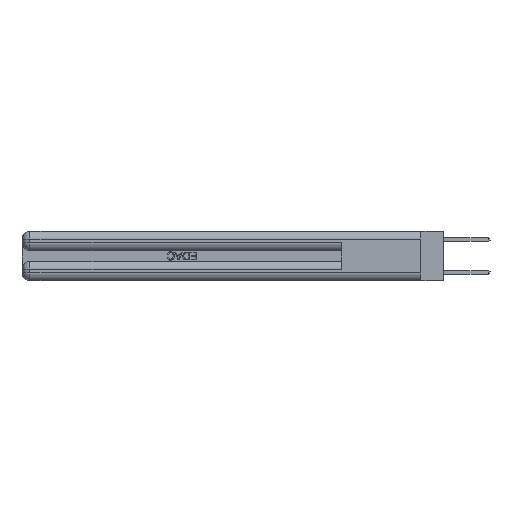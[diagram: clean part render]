
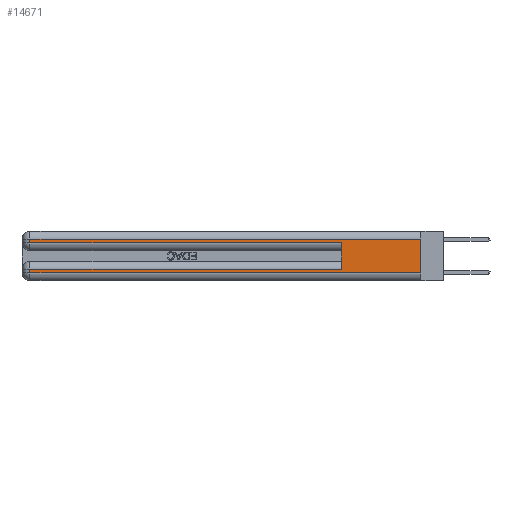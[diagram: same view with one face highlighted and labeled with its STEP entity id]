
A CAD part, left-side view. The second image highlights one B-rep face of the part: STEP entity #14671.
In plain terms, the highlighted planar face has unit normal (-1, 0, 0).
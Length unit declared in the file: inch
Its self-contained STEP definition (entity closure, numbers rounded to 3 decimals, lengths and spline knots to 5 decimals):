
#232 = CARTESIAN_POINT ( 'NONE',  ( 0., 0., 0.31 ) ) ;
#868 = CARTESIAN_POINT ( 'NONE',  ( 0., 0., 0.37 ) ) ;
#1439 = CARTESIAN_POINT ( 'NONE',  ( 0., 0.6, 0.145 ) ) ;
#1994 = CARTESIAN_POINT ( 'NONE',  ( 0., 2.94, 0.37 ) ) ;
#2072 = ORIENTED_EDGE ( 'NONE', *, *, #24333, .T. ) ;
#3748 = DIRECTION ( 'NONE',  ( 1., 0., 0. ) ) ;
#3786 = DIRECTION ( 'NONE',  ( 0., 1., 0. ) ) ;
#4033 = VECTOR ( 'NONE', #19386, 39.37008 ) ;
#4073 = VECTOR ( 'NONE', #12754, 39.37008 ) ;
#4190 = CARTESIAN_POINT ( 'NONE',  ( 0., 0.6, 0.285 ) ) ;
#4541 = VERTEX_POINT ( 'NONE', #232 ) ;
#4792 = EDGE_CURVE ( 'NONE', #25713, #32204, #33472, .T. ) ;
#4947 = CARTESIAN_POINT ( 'NONE',  ( 0., 0., 0.285 ) ) ;
#5174 = VERTEX_POINT ( 'NONE', #31147 ) ;
#5630 = FACE_OUTER_BOUND ( 'NONE', #18114, .T. ) ;
#5877 = LINE ( 'NONE', #23058, #18898 ) ;
#6047 = CARTESIAN_POINT ( 'NONE',  ( 0., 2.94, 0.37 ) ) ;
#7306 = ORIENTED_EDGE ( 'NONE', *, *, #11483, .T. ) ;
#7580 = DIRECTION ( 'NONE',  ( 0., 0., -1. ) ) ;
#7669 = CARTESIAN_POINT ( 'NONE',  ( 0., 2.94, 0.06 ) ) ;
#7971 = ORIENTED_EDGE ( 'NONE', *, *, #13333, .T. ) ;
#8860 = DIRECTION ( 'NONE',  ( 0., 0., -1. ) ) ;
#9326 = LINE ( 'NONE', #4947, #30485 ) ;
#9465 = CARTESIAN_POINT ( 'NONE',  ( 0., 0., 0.06 ) ) ;
#10545 = LINE ( 'NONE', #9465, #24324 ) ;
#10595 = ORIENTED_EDGE ( 'NONE', *, *, #23652, .T. ) ;
#11440 = ORIENTED_EDGE ( 'NONE', *, *, #23286, .T. ) ;
#11483 = EDGE_CURVE ( 'NONE', #26259, #22900, #30079, .T. ) ;
#11802 = AXIS2_PLACEMENT_3D ( 'NONE', #868, #3748, #23136 ) ;
#11980 = VECTOR ( 'NONE', #7580, 39.37008 ) ;
#12278 = DIRECTION ( 'NONE',  ( 0., -1., 0. ) ) ;
#12754 = DIRECTION ( 'NONE',  ( 0., 0., 1. ) ) ;
#13333 = EDGE_CURVE ( 'NONE', #33109, #18102, #10545, .T. ) ;
#14671 = ADVANCED_FACE ( 'NONE', ( #5630 ), #17615, .F. ) ;
#15400 = VECTOR ( 'NONE', #8860, 39.37008 ) ;
#15519 = EDGE_CURVE ( 'NONE', #25713, #5174, #17287, .T. ) ;
#17287 = LINE ( 'NONE', #34120, #22885 ) ;
#17615 = PLANE ( 'NONE',  #11802 ) ;
#18102 = VERTEX_POINT ( 'NONE', #20254 ) ;
#18114 = EDGE_LOOP ( 'NONE', ( #21432, #10595, #7306, #11440, #27233, #25093, #2072, #7971 ) ) ;
#18898 = VECTOR ( 'NONE', #3786, 39.37008 ) ;
#18994 = CARTESIAN_POINT ( 'NONE',  ( 0., 0.6, 0.085 ) ) ;
#19386 = DIRECTION ( 'NONE',  ( 0., 0., -1. ) ) ;
#20254 = CARTESIAN_POINT ( 'NONE',  ( 0., 0., 0.06 ) ) ;
#21432 = ORIENTED_EDGE ( 'NONE', *, *, #25056, .F. ) ;
#21545 = DIRECTION ( 'NONE',  ( 0., -1., 0. ) ) ;
#22885 = VECTOR ( 'NONE', #33779, 39.37008 ) ;
#22900 = VERTEX_POINT ( 'NONE', #30713 ) ;
#23058 = CARTESIAN_POINT ( 'NONE',  ( 0., 0., 0.31 ) ) ;
#23136 = DIRECTION ( 'NONE',  ( 0., 0., -1. ) ) ;
#23286 = EDGE_CURVE ( 'NONE', #22900, #32204, #9326, .T. ) ;
#23652 = EDGE_CURVE ( 'NONE', #4541, #26259, #5877, .T. ) ;
#24324 = VECTOR ( 'NONE', #12278, 39.37008 ) ;
#24333 = EDGE_CURVE ( 'NONE', #5174, #33109, #26617, .T. ) ;
#24585 = CARTESIAN_POINT ( 'NONE',  ( 0., 2.94, 0.31 ) ) ;
#25056 = EDGE_CURVE ( 'NONE', #4541, #18102, #32583, .T. ) ;
#25093 = ORIENTED_EDGE ( 'NONE', *, *, #15519, .T. ) ;
#25713 = VERTEX_POINT ( 'NONE', #18994 ) ;
#26259 = VERTEX_POINT ( 'NONE', #24585 ) ;
#26617 = LINE ( 'NONE', #1994, #11980 ) ;
#27233 = ORIENTED_EDGE ( 'NONE', *, *, #4792, .F. ) ;
#30079 = LINE ( 'NONE', #6047, #15400 ) ;
#30485 = VECTOR ( 'NONE', #21545, 39.37008 ) ;
#30713 = CARTESIAN_POINT ( 'NONE',  ( 0., 2.94, 0.285 ) ) ;
#31147 = CARTESIAN_POINT ( 'NONE',  ( 0., 2.94, 0.085 ) ) ;
#32204 = VERTEX_POINT ( 'NONE', #4190 ) ;
#32583 = LINE ( 'NONE', #33076, #4033 ) ;
#33076 = CARTESIAN_POINT ( 'NONE',  ( 0., 0., 0.37 ) ) ;
#33109 = VERTEX_POINT ( 'NONE', #7669 ) ;
#33472 = LINE ( 'NONE', #1439, #4073 ) ;
#33779 = DIRECTION ( 'NONE',  ( 0., 1., 0. ) ) ;
#34120 = CARTESIAN_POINT ( 'NONE',  ( 0., 0., 0.085 ) ) ;
